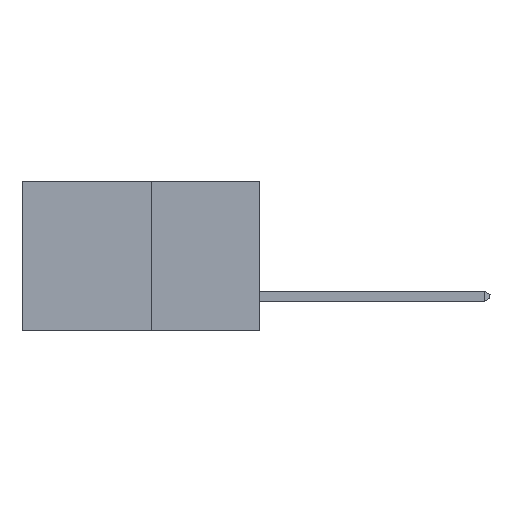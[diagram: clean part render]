
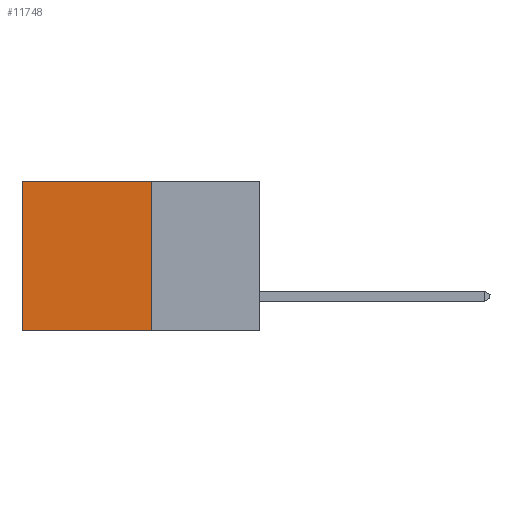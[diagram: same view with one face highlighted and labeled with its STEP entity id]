
A CAD part, left-side view. The second image highlights one B-rep face of the part: STEP entity #11748.
In plain terms, the highlighted planar face has unit normal (-1, 0, 0).
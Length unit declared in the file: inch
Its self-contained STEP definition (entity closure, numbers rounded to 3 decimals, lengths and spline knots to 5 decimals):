
#1088 = VERTEX_POINT ( 'NONE', #10647 ) ;
#1485 = CARTESIAN_POINT ( 'NONE',  ( 0.277, 0.59, -0.37 ) ) ;
#1594 = CARTESIAN_POINT ( 'NONE',  ( 0.277, 0.27, -0.37 ) ) ;
#1901 = ORIENTED_EDGE ( 'NONE', *, *, #13032, .T. ) ;
#2459 = LINE ( 'NONE', #1485, #8038 ) ;
#3297 = CARTESIAN_POINT ( 'NONE',  ( 0.277, 0.59, -0.37 ) ) ;
#3951 = EDGE_LOOP ( 'NONE', ( #13636, #5810, #5091, #1901 ) ) ;
#4686 = VECTOR ( 'NONE', #11393, 39.37008 ) ;
#4881 = VERTEX_POINT ( 'NONE', #3297 ) ;
#5091 = ORIENTED_EDGE ( 'NONE', *, *, #10459, .F. ) ;
#5810 = ORIENTED_EDGE ( 'NONE', *, *, #6448, .F. ) ;
#6345 = LINE ( 'NONE', #11597, #11227 ) ;
#6362 = EDGE_CURVE ( 'NONE', #13525, #4881, #2459, .T. ) ;
#6448 = EDGE_CURVE ( 'NONE', #1088, #4881, #9086, .T. ) ;
#6863 = DIRECTION ( 'NONE',  ( 0., 0., -1. ) ) ;
#7158 = DIRECTION ( 'NONE',  ( 0., 0., -1. ) ) ;
#7403 = CARTESIAN_POINT ( 'NONE',  ( 0.277, 0.27, 0. ) ) ;
#7428 = VERTEX_POINT ( 'NONE', #7403 ) ;
#7703 = VECTOR ( 'NONE', #9369, 39.37008 ) ;
#7941 = CARTESIAN_POINT ( 'NONE',  ( 0.277, 0.59, 0. ) ) ;
#8038 = VECTOR ( 'NONE', #7158, 39.37008 ) ;
#8773 = AXIS2_PLACEMENT_3D ( 'NONE', #12047, #13056, #6863 ) ;
#8932 = PLANE ( 'NONE',  #8773 ) ;
#9086 = LINE ( 'NONE', #1594, #7703 ) ;
#9369 = DIRECTION ( 'NONE',  ( 0., 1., 0. ) ) ;
#9563 = DIRECTION ( 'NONE',  ( 0., 1., 0. ) ) ;
#10459 = EDGE_CURVE ( 'NONE', #7428, #1088, #12696, .T. ) ;
#10647 = CARTESIAN_POINT ( 'NONE',  ( 0.277, 0.27, -0.37 ) ) ;
#11227 = VECTOR ( 'NONE', #9563, 39.37008 ) ;
#11393 = DIRECTION ( 'NONE',  ( 0., 0., -1. ) ) ;
#11597 = CARTESIAN_POINT ( 'NONE',  ( 0.277, 0.27, 0. ) ) ;
#11745 = FACE_OUTER_BOUND ( 'NONE', #3951, .T. ) ;
#11748 = ADVANCED_FACE ( 'NONE', ( #11745 ), #8932, .F. ) ;
#12047 = CARTESIAN_POINT ( 'NONE',  ( 0.277, 0.27, -0.37 ) ) ;
#12696 = LINE ( 'NONE', #13371, #4686 ) ;
#13032 = EDGE_CURVE ( 'NONE', #7428, #13525, #6345, .T. ) ;
#13056 = DIRECTION ( 'NONE',  ( 1., 0., 0. ) ) ;
#13371 = CARTESIAN_POINT ( 'NONE',  ( 0.277, 0.27, -0.37 ) ) ;
#13525 = VERTEX_POINT ( 'NONE', #7941 ) ;
#13636 = ORIENTED_EDGE ( 'NONE', *, *, #6362, .T. ) ;
